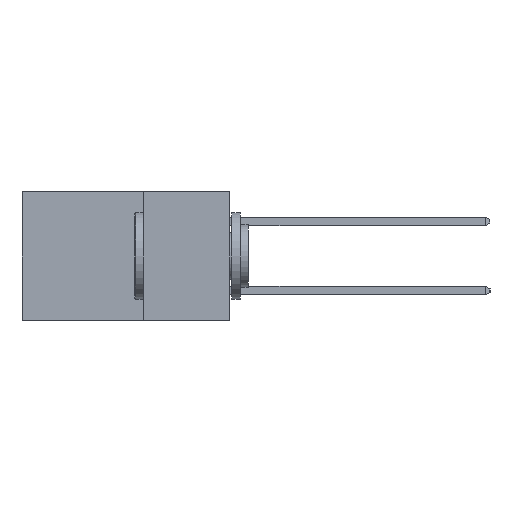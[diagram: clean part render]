
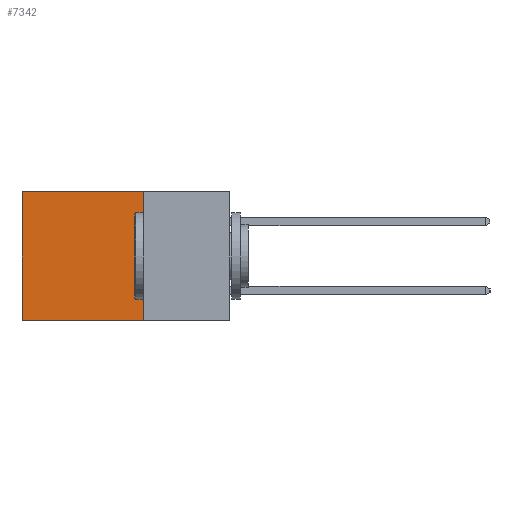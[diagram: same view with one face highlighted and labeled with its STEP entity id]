
A CAD part, left-side view. The second image highlights one B-rep face of the part: STEP entity #7342.
In plain terms, the highlighted planar face has unit normal (-1, 0, 0).
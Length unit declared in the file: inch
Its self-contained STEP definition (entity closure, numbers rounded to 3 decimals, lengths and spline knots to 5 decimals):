
#976 = VECTOR ( 'NONE', #12968, 39.37008 ) ;
#1299 = ORIENTED_EDGE ( 'NONE', *, *, #13568, .T. ) ;
#1381 = LINE ( 'NONE', #17207, #18477 ) ;
#1666 = LINE ( 'NONE', #12195, #14396 ) ;
#1892 = CARTESIAN_POINT ( 'NONE',  ( 0.2615, 0.25, 0. ) ) ;
#1979 = LINE ( 'NONE', #17493, #18550 ) ;
#3692 = VERTEX_POINT ( 'NONE', #12948 ) ;
#4343 = EDGE_LOOP ( 'NONE', ( #1299, #11537, #16546, #20463 ) ) ;
#4430 = AXIS2_PLACEMENT_3D ( 'NONE', #12328, #11547, #11486 ) ;
#5179 = CARTESIAN_POINT ( 'NONE',  ( 0.2615, 0.6, 0. ) ) ;
#5623 = EDGE_CURVE ( 'NONE', #18127, #11085, #1666, .T. ) ;
#5625 = DIRECTION ( 'NONE',  ( 0., 0., -1. ) ) ;
#7342 = ADVANCED_FACE ( 'NONE', ( #8400 ), #11672, .F. ) ;
#7627 = CARTESIAN_POINT ( 'NONE',  ( 0.2615, 0.6, -0.37 ) ) ;
#8400 = FACE_OUTER_BOUND ( 'NONE', #4343, .T. ) ;
#10869 = EDGE_CURVE ( 'NONE', #3692, #17848, #14221, .T. ) ;
#10938 = DIRECTION ( 'NONE',  ( 0., 0., -1. ) ) ;
#11085 = VERTEX_POINT ( 'NONE', #5179 ) ;
#11306 = CARTESIAN_POINT ( 'NONE',  ( 0.2615, 0.25, -0.37 ) ) ;
#11486 = DIRECTION ( 'NONE',  ( 0., 0., -1. ) ) ;
#11537 = ORIENTED_EDGE ( 'NONE', *, *, #10869, .F. ) ;
#11547 = DIRECTION ( 'NONE',  ( 1., 0., 0. ) ) ;
#11672 = PLANE ( 'NONE',  #4430 ) ;
#11769 = EDGE_CURVE ( 'NONE', #18127, #3692, #1979, .T. ) ;
#12166 = DIRECTION ( 'NONE',  ( 0., 1., 0. ) ) ;
#12195 = CARTESIAN_POINT ( 'NONE',  ( 0.2615, 0.25, 0. ) ) ;
#12328 = CARTESIAN_POINT ( 'NONE',  ( 0.2615, 0.25, -0.37 ) ) ;
#12948 = CARTESIAN_POINT ( 'NONE',  ( 0.2615, 0.25, -0.37 ) ) ;
#12968 = DIRECTION ( 'NONE',  ( 0., 1., 0. ) ) ;
#13568 = EDGE_CURVE ( 'NONE', #11085, #17848, #1381, .T. ) ;
#14221 = LINE ( 'NONE', #11306, #976 ) ;
#14396 = VECTOR ( 'NONE', #12166, 39.37008 ) ;
#16546 = ORIENTED_EDGE ( 'NONE', *, *, #11769, .F. ) ;
#17207 = CARTESIAN_POINT ( 'NONE',  ( 0.2615, 0.6, -0.37 ) ) ;
#17493 = CARTESIAN_POINT ( 'NONE',  ( 0.2615, 0.25, -0.37 ) ) ;
#17848 = VERTEX_POINT ( 'NONE', #7627 ) ;
#18127 = VERTEX_POINT ( 'NONE', #1892 ) ;
#18477 = VECTOR ( 'NONE', #5625, 39.37008 ) ;
#18550 = VECTOR ( 'NONE', #10938, 39.37008 ) ;
#20463 = ORIENTED_EDGE ( 'NONE', *, *, #5623, .T. ) ;
